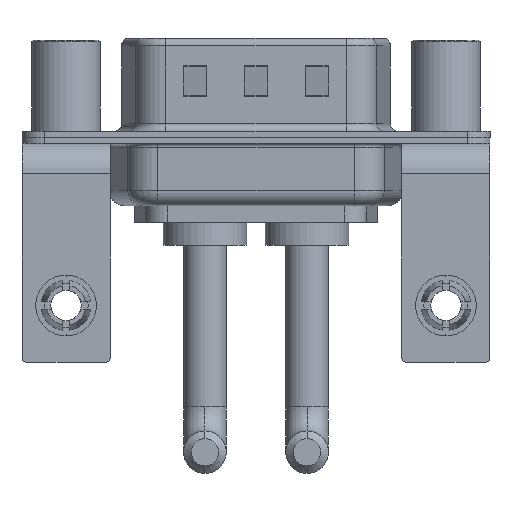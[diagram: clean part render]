
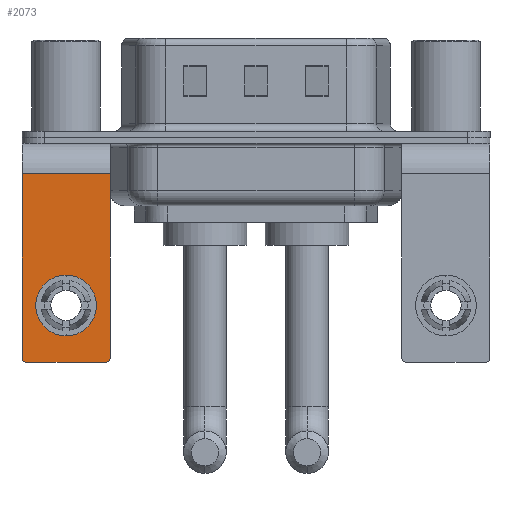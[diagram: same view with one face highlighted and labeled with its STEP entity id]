
A CAD part, front view. The second image highlights one B-rep face of the part: STEP entity #2073.
In plain terms, the highlighted planar face has unit normal (0, -1, 0).
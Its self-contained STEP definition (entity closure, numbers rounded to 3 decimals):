
#112 = FACE_OUTER_BOUND ( 'NONE', #5492, .T. ) ;
#412 = EDGE_LOOP ( 'NONE', ( #8263, #10669 ) ) ;
#484 = CARTESIAN_POINT ( 'NONE',  ( -2.9, -6.25, -2.4 ) ) ;
#545 = DIRECTION ( 'NONE',  ( -1., 0., 0. ) ) ;
#711 = CARTESIAN_POINT ( 'NONE',  ( 0., -6.25, -9.07 ) ) ;
#959 = CARTESIAN_POINT ( 'NONE',  ( -2.65, -6.25, -14.55 ) ) ;
#1241 = CARTESIAN_POINT ( 'NONE',  ( -2.9, -6.25, -2.4 ) ) ;
#1745 = PLANE ( 'NONE',  #17732 ) ;
#1762 = DIRECTION ( 'NONE',  ( 0., 0., 1. ) ) ;
#2028 = DIRECTION ( 'NONE',  ( 0., 1., 0. ) ) ;
#2073 = ADVANCED_FACE ( 'NONE', ( #15502, #112 ), #1745, .F. ) ;
#2274 = VERTEX_POINT ( 'NONE', #14232 ) ;
#2332 = DIRECTION ( 'NONE',  ( 0., 0., 1. ) ) ;
#2717 = CIRCLE ( 'NONE', #10832, 0.25 ) ;
#3010 = DIRECTION ( 'NONE',  ( 0., 0., 1. ) ) ;
#3107 = LINE ( 'NONE', #10359, #8445 ) ;
#3297 = DIRECTION ( 'NONE',  ( 0., 0., -1. ) ) ;
#3458 = EDGE_CURVE ( 'NONE', #4749, #5465, #9686, .T. ) ;
#3927 = VECTOR ( 'NONE', #10370, 1000. ) ;
#4067 = LINE ( 'NONE', #8142, #15260 ) ;
#4458 = EDGE_CURVE ( 'NONE', #2274, #15672, #15761, .T. ) ;
#4563 = ORIENTED_EDGE ( 'NONE', *, *, #6620, .F. ) ;
#4648 = LINE ( 'NONE', #10184, #3927 ) ;
#4749 = VERTEX_POINT ( 'NONE', #13512 ) ;
#4848 = LINE ( 'NONE', #484, #9627 ) ;
#5048 = DIRECTION ( 'NONE',  ( 0., -1., 0. ) ) ;
#5465 = VERTEX_POINT ( 'NONE', #13584 ) ;
#5492 = EDGE_LOOP ( 'NONE', ( #13233, #8867, #4563, #6487, #13575, #12125 ) ) ;
#6487 = ORIENTED_EDGE ( 'NONE', *, *, #3458, .T. ) ;
#6620 = EDGE_CURVE ( 'NONE', #4749, #10381, #4067, .T. ) ;
#7973 = AXIS2_PLACEMENT_3D ( 'NONE', #12100, #2028, #12007 ) ;
#8142 = CARTESIAN_POINT ( 'NONE',  ( 2.9, -6.25, -14.8 ) ) ;
#8263 = ORIENTED_EDGE ( 'NONE', *, *, #4458, .T. ) ;
#8445 = VECTOR ( 'NONE', #545, 1000. ) ;
#8479 = EDGE_CURVE ( 'NONE', #15672, #2274, #11362, .T. ) ;
#8867 = ORIENTED_EDGE ( 'NONE', *, *, #11599, .T. ) ;
#9018 = CARTESIAN_POINT ( 'NONE',  ( -2.65, -6.25, -14.8 ) ) ;
#9308 = DIRECTION ( 'NONE',  ( 0., 0., 1. ) ) ;
#9477 = EDGE_CURVE ( 'NONE', #15759, #11609, #3107, .T. ) ;
#9627 = VECTOR ( 'NONE', #3297, 1000. ) ;
#9686 = CIRCLE ( 'NONE', #14294, 0.25 ) ;
#10184 = CARTESIAN_POINT ( 'NONE',  ( 2.9, -6.25, -2.4 ) ) ;
#10326 = EDGE_CURVE ( 'NONE', #11609, #12938, #4848, .T. ) ;
#10359 = CARTESIAN_POINT ( 'NONE',  ( 2.9, -6.25, -2.4 ) ) ;
#10370 = DIRECTION ( 'NONE',  ( 0., 0., -1. ) ) ;
#10381 = VERTEX_POINT ( 'NONE', #9018 ) ;
#10669 = ORIENTED_EDGE ( 'NONE', *, *, #8479, .T. ) ;
#10773 = CARTESIAN_POINT ( 'NONE',  ( -2.9, -6.25, -14.55 ) ) ;
#10832 = AXIS2_PLACEMENT_3D ( 'NONE', #959, #5048, #2332 ) ;
#11362 = CIRCLE ( 'NONE', #11642, 2. ) ;
#11599 = EDGE_CURVE ( 'NONE', #12938, #10381, #2717, .T. ) ;
#11609 = VERTEX_POINT ( 'NONE', #1241 ) ;
#11642 = AXIS2_PLACEMENT_3D ( 'NONE', #14169, #15873, #1762 ) ;
#12007 = DIRECTION ( 'NONE',  ( 0., 0., 1. ) ) ;
#12100 = CARTESIAN_POINT ( 'NONE',  ( 0., -6.25, -11.07 ) ) ;
#12125 = ORIENTED_EDGE ( 'NONE', *, *, #9477, .T. ) ;
#12938 = VERTEX_POINT ( 'NONE', #10773 ) ;
#13233 = ORIENTED_EDGE ( 'NONE', *, *, #10326, .T. ) ;
#13512 = CARTESIAN_POINT ( 'NONE',  ( 2.65, -6.25, -14.8 ) ) ;
#13575 = ORIENTED_EDGE ( 'NONE', *, *, #13789, .F. ) ;
#13584 = CARTESIAN_POINT ( 'NONE',  ( 2.9, -6.25, -14.55 ) ) ;
#13668 = DIRECTION ( 'NONE',  ( -1., 0., 0. ) ) ;
#13789 = EDGE_CURVE ( 'NONE', #15759, #5465, #4648, .T. ) ;
#14061 = DIRECTION ( 'NONE',  ( 0., 1., 0. ) ) ;
#14169 = CARTESIAN_POINT ( 'NONE',  ( 0., -6.25, -11.07 ) ) ;
#14232 = CARTESIAN_POINT ( 'NONE',  ( 0., -6.25, -13.07 ) ) ;
#14294 = AXIS2_PLACEMENT_3D ( 'NONE', #14542, #17347, #9308 ) ;
#14542 = CARTESIAN_POINT ( 'NONE',  ( 2.65, -6.25, -14.55 ) ) ;
#15260 = VECTOR ( 'NONE', #13668, 1000. ) ;
#15502 = FACE_BOUND ( 'NONE', #412, .T. ) ;
#15672 = VERTEX_POINT ( 'NONE', #711 ) ;
#15759 = VERTEX_POINT ( 'NONE', #15926 ) ;
#15761 = CIRCLE ( 'NONE', #7973, 2. ) ;
#15873 = DIRECTION ( 'NONE',  ( 0., 1., 0. ) ) ;
#15926 = CARTESIAN_POINT ( 'NONE',  ( 2.9, -6.25, -2.4 ) ) ;
#16676 = CARTESIAN_POINT ( 'NONE',  ( 2.9, -6.25, -2.4 ) ) ;
#17347 = DIRECTION ( 'NONE',  ( 0., -1., 0. ) ) ;
#17732 = AXIS2_PLACEMENT_3D ( 'NONE', #16676, #14061, #3010 ) ;
